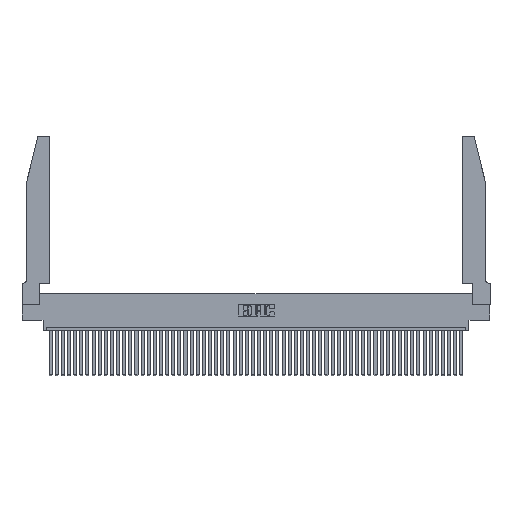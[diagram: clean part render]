
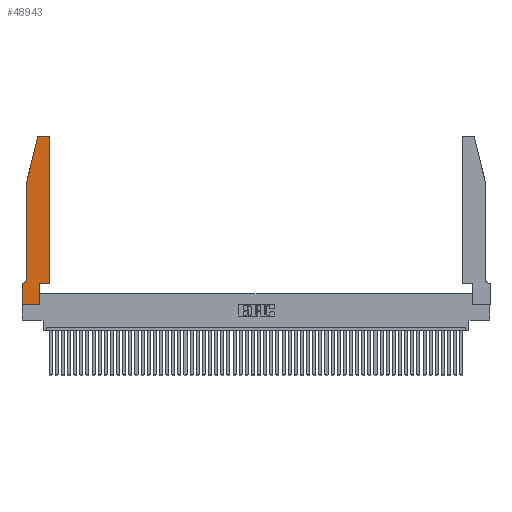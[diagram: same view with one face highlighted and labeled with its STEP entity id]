
A CAD part, top view. The second image highlights one B-rep face of the part: STEP entity #48943.
In plain terms, the highlighted planar face has unit normal (0, 0, 1).
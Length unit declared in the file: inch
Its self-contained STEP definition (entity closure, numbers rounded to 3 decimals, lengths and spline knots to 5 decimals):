
#642 = VERTEX_POINT ( 'NONE', #36980 ) ;
#823 = VECTOR ( 'NONE', #34067, 39.37008 ) ;
#1047 = CARTESIAN_POINT ( 'NONE',  ( 0., 0., 0.37 ) ) ;
#1308 = EDGE_CURVE ( 'NONE', #642, #11872, #19926, .T. ) ;
#1476 = CARTESIAN_POINT ( 'NONE',  ( 0.4505, 0.35, 0.37 ) ) ;
#1997 = CARTESIAN_POINT ( 'NONE',  ( 0.0755, 0.42, 0.37 ) ) ;
#2099 = ORIENTED_EDGE ( 'NONE', *, *, #43149, .T. ) ;
#2128 = ORIENTED_EDGE ( 'NONE', *, *, #4987, .T. ) ;
#2240 = CARTESIAN_POINT ( 'NONE',  ( 0.2605, 2.75, 0.37 ) ) ;
#3079 = CARTESIAN_POINT ( 'NONE',  ( 0.2865, 0., 0.37 ) ) ;
#3198 = CARTESIAN_POINT ( 'NONE',  ( 0.0755, 2., 0.37 ) ) ;
#3787 = VECTOR ( 'NONE', #30566, 39.37008 ) ;
#4541 = CARTESIAN_POINT ( 'NONE',  ( 0., 0.35, 0.37 ) ) ;
#4987 = EDGE_CURVE ( 'NONE', #50336, #43063, #40546, .T. ) ;
#5150 = DIRECTION ( 'NONE',  ( 1., 0., 0. ) ) ;
#5519 = ORIENTED_EDGE ( 'NONE', *, *, #41888, .T. ) ;
#6694 = CARTESIAN_POINT ( 'NONE',  ( 0.2865, 0.35, 0.37 ) ) ;
#7165 = CARTESIAN_POINT ( 'NONE',  ( 0.284, 2.72, 0.37 ) ) ;
#7354 = VECTOR ( 'NONE', #42784, 39.37008 ) ;
#7786 = CARTESIAN_POINT ( 'NONE',  ( 0.0055, 0.35, 0.37 ) ) ;
#8086 = VECTOR ( 'NONE', #48335, 39.37008 ) ;
#8087 = VERTEX_POINT ( 'NONE', #13927 ) ;
#8367 = CARTESIAN_POINT ( 'NONE',  ( 0.0755, 2., 0.37 ) ) ;
#9405 = CARTESIAN_POINT ( 'NONE',  ( 0.4505, 0.35, 0.37 ) ) ;
#11367 = LINE ( 'NONE', #37793, #21995 ) ;
#11747 = LINE ( 'NONE', #8367, #823 ) ;
#11872 = VERTEX_POINT ( 'NONE', #28801 ) ;
#12870 = LINE ( 'NONE', #38029, #42665 ) ;
#12921 = DIRECTION ( 'NONE',  ( 1., 0., 0. ) ) ;
#12930 = CARTESIAN_POINT ( 'NONE',  ( 0.0055, 0.42, 0.37 ) ) ;
#13927 = CARTESIAN_POINT ( 'NONE',  ( 0.4505, 2.72, 0.37 ) ) ;
#14235 = ORIENTED_EDGE ( 'NONE', *, *, #23061, .T. ) ;
#14616 = VERTEX_POINT ( 'NONE', #46961 ) ;
#15133 = CIRCLE ( 'NONE', #35764, 0.03 ) ;
#15286 = DIRECTION ( 'NONE',  ( 1., 0., 0. ) ) ;
#15567 = VERTEX_POINT ( 'NONE', #3079 ) ;
#16642 = VECTOR ( 'NONE', #5150, 39.37008 ) ;
#17548 = DIRECTION ( 'NONE',  ( 1., 0., 0. ) ) ;
#17799 = DIRECTION ( 'NONE',  ( 0., 1., 0. ) ) ;
#18033 = DIRECTION ( 'NONE',  ( 0., 0., -1. ) ) ;
#18616 = CARTESIAN_POINT ( 'NONE',  ( 0.2865, 0.35, 0.37 ) ) ;
#19926 = LINE ( 'NONE', #2240, #7354 ) ;
#20611 = VERTEX_POINT ( 'NONE', #1047 ) ;
#20986 = ORIENTED_EDGE ( 'NONE', *, *, #21534, .T. ) ;
#21534 = EDGE_CURVE ( 'NONE', #14616, #50336, #11747, .T. ) ;
#21995 = VECTOR ( 'NONE', #17548, 39.37008 ) ;
#22811 = ORIENTED_EDGE ( 'NONE', *, *, #38959, .T. ) ;
#23061 = EDGE_CURVE ( 'NONE', #43063, #39347, #26080, .T. ) ;
#23261 = ORIENTED_EDGE ( 'NONE', *, *, #23874, .T. ) ;
#23874 = EDGE_CURVE ( 'NONE', #39347, #43967, #50627, .T. ) ;
#24136 = CIRCLE ( 'NONE', #43227, 0.03 ) ;
#24745 = EDGE_CURVE ( 'NONE', #20611, #15567, #11367, .T. ) ;
#26080 = CIRCLE ( 'NONE', #31301, 0.07 ) ;
#28801 = CARTESIAN_POINT ( 'NONE',  ( 0.284, 2.75, 0.37 ) ) ;
#30338 = DIRECTION ( 'NONE',  ( -1., 0., 0. ) ) ;
#30566 = DIRECTION ( 'NONE',  ( 0., -1., 0. ) ) ;
#31301 = AXIS2_PLACEMENT_3D ( 'NONE', #12930, #18033, #30338 ) ;
#31640 = DIRECTION ( 'NONE',  ( 0., 0., 1. ) ) ;
#32160 = ORIENTED_EDGE ( 'NONE', *, *, #44856, .T. ) ;
#34067 = DIRECTION ( 'NONE',  ( -0.239, -0.971, 0. ) ) ;
#34190 = VERTEX_POINT ( 'NONE', #6694 ) ;
#35158 = VERTEX_POINT ( 'NONE', #1476 ) ;
#35525 = DIRECTION ( 'NONE',  ( -1., 0., 0. ) ) ;
#35764 = AXIS2_PLACEMENT_3D ( 'NONE', #41248, #40926, #12921 ) ;
#36786 = ORIENTED_EDGE ( 'NONE', *, *, #1308, .T. ) ;
#36980 = CARTESIAN_POINT ( 'NONE',  ( 0.4205, 2.75, 0.37 ) ) ;
#37248 = VECTOR ( 'NONE', #47507, 39.37008 ) ;
#37793 = CARTESIAN_POINT ( 'NONE',  ( 0., 0., 0.37 ) ) ;
#38029 = CARTESIAN_POINT ( 'NONE',  ( 0.4505, 0.35, 0.37 ) ) ;
#38154 = ORIENTED_EDGE ( 'NONE', *, *, #47999, .T. ) ;
#38959 = EDGE_CURVE ( 'NONE', #15567, #34190, #45220, .T. ) ;
#39347 = VERTEX_POINT ( 'NONE', #7786 ) ;
#40546 = LINE ( 'NONE', #50391, #3787 ) ;
#40692 = PLANE ( 'NONE',  #51754 ) ;
#40926 = DIRECTION ( 'NONE',  ( 0., 0., 1. ) ) ;
#41177 = VECTOR ( 'NONE', #35525, 39.37008 ) ;
#41248 = CARTESIAN_POINT ( 'NONE',  ( 0.4205, 2.72, 0.37 ) ) ;
#41888 = EDGE_CURVE ( 'NONE', #11872, #14616, #24136, .T. ) ;
#42665 = VECTOR ( 'NONE', #17799, 39.37008 ) ;
#42784 = DIRECTION ( 'NONE',  ( -1., 0., 0. ) ) ;
#43063 = VERTEX_POINT ( 'NONE', #1997 ) ;
#43149 = EDGE_CURVE ( 'NONE', #43967, #20611, #48055, .T. ) ;
#43227 = AXIS2_PLACEMENT_3D ( 'NONE', #7165, #31640, #15286 ) ;
#43967 = VERTEX_POINT ( 'NONE', #49952 ) ;
#44675 = DIRECTION ( 'NONE',  ( 0., 0., 1. ) ) ;
#44856 = EDGE_CURVE ( 'NONE', #8087, #642, #15133, .T. ) ;
#45220 = LINE ( 'NONE', #18616, #8086 ) ;
#45559 = EDGE_LOOP ( 'NONE', ( #36786, #5519, #20986, #2128, #14235, #23261, #2099, #49388, #22811, #38154, #48721, #32160 ) ) ;
#46961 = CARTESIAN_POINT ( 'NONE',  ( 0.25487, 2.72718, 0.37 ) ) ;
#47490 = CARTESIAN_POINT ( 'NONE',  ( 0.0755, 0.35, 0.37 ) ) ;
#47507 = DIRECTION ( 'NONE',  ( 0., -1., 0. ) ) ;
#47999 = EDGE_CURVE ( 'NONE', #34190, #35158, #48919, .T. ) ;
#48055 = LINE ( 'NONE', #51567, #37248 ) ;
#48335 = DIRECTION ( 'NONE',  ( 0., 1., 0. ) ) ;
#48721 = ORIENTED_EDGE ( 'NONE', *, *, #52164, .T. ) ;
#48759 = DIRECTION ( 'NONE',  ( 1., 0., 0. ) ) ;
#48919 = LINE ( 'NONE', #9405, #16642 ) ;
#48943 = ADVANCED_FACE ( 'NONE', ( #50715 ), #40692, .T. ) ;
#49388 = ORIENTED_EDGE ( 'NONE', *, *, #24745, .T. ) ;
#49952 = CARTESIAN_POINT ( 'NONE',  ( 0., 0.35, 0.37 ) ) ;
#50336 = VERTEX_POINT ( 'NONE', #3198 ) ;
#50391 = CARTESIAN_POINT ( 'NONE',  ( 0.0755, 2., 0.37 ) ) ;
#50627 = LINE ( 'NONE', #47490, #41177 ) ;
#50715 = FACE_OUTER_BOUND ( 'NONE', #45559, .T. ) ;
#51567 = CARTESIAN_POINT ( 'NONE',  ( 0., 0., 0.37 ) ) ;
#51754 = AXIS2_PLACEMENT_3D ( 'NONE', #4541, #44675, #48759 ) ;
#52164 = EDGE_CURVE ( 'NONE', #35158, #8087, #12870, .T. ) ;
